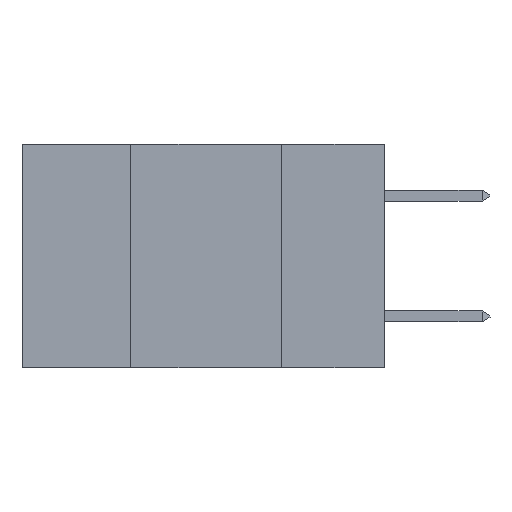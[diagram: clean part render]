
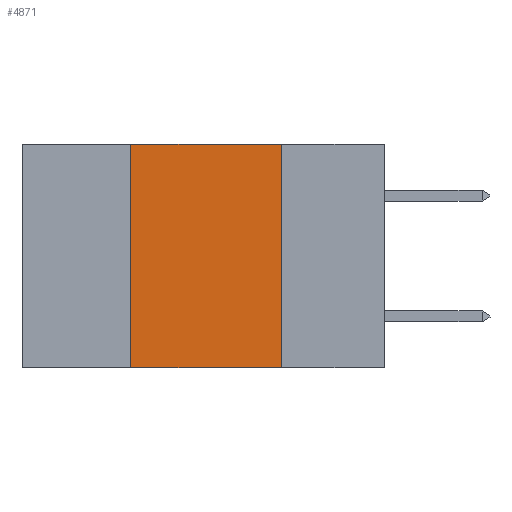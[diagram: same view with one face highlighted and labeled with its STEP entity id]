
A CAD part, left-side view. The second image highlights one B-rep face of the part: STEP entity #4871.
In plain terms, the highlighted planar face has unit normal (-1, 0, 0).
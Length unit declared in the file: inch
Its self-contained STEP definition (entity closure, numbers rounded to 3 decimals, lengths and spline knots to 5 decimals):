
#178 = VERTEX_POINT ( 'NONE', #1802 ) ;
#1438 = VERTEX_POINT ( 'NONE', #18476 ) ;
#1443 = CARTESIAN_POINT ( 'NONE',  ( 0., 0.6, 0. ) ) ;
#1802 = CARTESIAN_POINT ( 'NONE',  ( 0., 0.42, 0. ) ) ;
#2023 = EDGE_CURVE ( 'NONE', #11006, #20083, #9775, .T. ) ;
#2457 = CARTESIAN_POINT ( 'NONE',  ( 0., 0.42, 0. ) ) ;
#2934 = ORIENTED_EDGE ( 'NONE', *, *, #18386, .F. ) ;
#3206 = DIRECTION ( 'NONE',  ( 0., 0., -1. ) ) ;
#3365 = CARTESIAN_POINT ( 'NONE',  ( 0., 0.42, -0.37 ) ) ;
#3495 = ORIENTED_EDGE ( 'NONE', *, *, #18554, .F. ) ;
#3609 = CARTESIAN_POINT ( 'NONE',  ( 0., 0.17, -0.37 ) ) ;
#4756 = ORIENTED_EDGE ( 'NONE', *, *, #2023, .T. ) ;
#4871 = ADVANCED_FACE ( 'NONE', ( #10159 ), #9883, .F. ) ;
#5873 = VECTOR ( 'NONE', #11442, 39.37008 ) ;
#7081 = DIRECTION ( 'NONE',  ( 0., 0., -1. ) ) ;
#7307 = LINE ( 'NONE', #17335, #15884 ) ;
#8048 = AXIS2_PLACEMENT_3D ( 'NONE', #1443, #13381, #3206 ) ;
#9775 = LINE ( 'NONE', #10426, #5873 ) ;
#9883 = PLANE ( 'NONE',  #8048 ) ;
#10159 = FACE_OUTER_BOUND ( 'NONE', #18471, .T. ) ;
#10426 = CARTESIAN_POINT ( 'NONE',  ( 0., 0.6, -0.37 ) ) ;
#11006 = VERTEX_POINT ( 'NONE', #3365 ) ;
#11442 = DIRECTION ( 'NONE',  ( 0., -1., 0. ) ) ;
#12671 = DIRECTION ( 'NONE',  ( 0., 0., 1. ) ) ;
#13381 = DIRECTION ( 'NONE',  ( 1., 0., 0. ) ) ;
#13436 = DIRECTION ( 'NONE',  ( 0., -1., 0. ) ) ;
#14370 = ORIENTED_EDGE ( 'NONE', *, *, #19704, .F. ) ;
#15643 = VECTOR ( 'NONE', #13436, 39.37008 ) ;
#15884 = VECTOR ( 'NONE', #7081, 39.37008 ) ;
#16361 = VECTOR ( 'NONE', #12671, 39.37008 ) ;
#17335 = CARTESIAN_POINT ( 'NONE',  ( 0., 0.17, 0. ) ) ;
#18386 = EDGE_CURVE ( 'NONE', #178, #1438, #20218, .T. ) ;
#18471 = EDGE_LOOP ( 'NONE', ( #3495, #2934, #14370, #4756 ) ) ;
#18476 = CARTESIAN_POINT ( 'NONE',  ( 0., 0.17, 0. ) ) ;
#18554 = EDGE_CURVE ( 'NONE', #1438, #20083, #7307, .T. ) ;
#19704 = EDGE_CURVE ( 'NONE', #11006, #178, #20904, .T. ) ;
#20083 = VERTEX_POINT ( 'NONE', #3609 ) ;
#20218 = LINE ( 'NONE', #20305, #15643 ) ;
#20305 = CARTESIAN_POINT ( 'NONE',  ( 0., 0.6, 0. ) ) ;
#20904 = LINE ( 'NONE', #2457, #16361 ) ;
